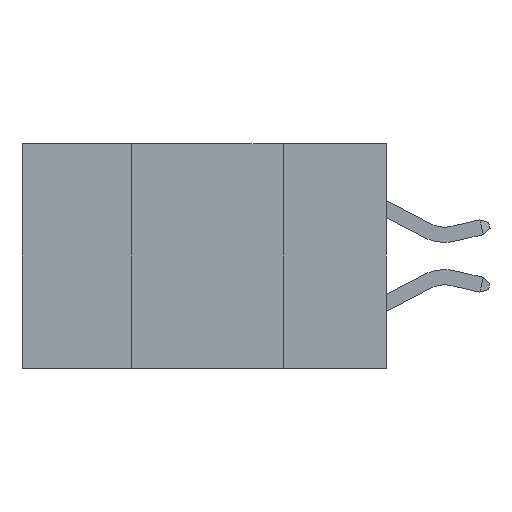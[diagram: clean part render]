
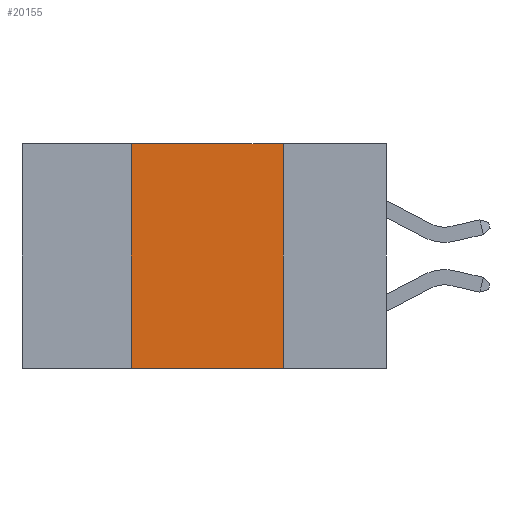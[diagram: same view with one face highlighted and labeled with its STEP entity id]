
A CAD part, left-side view. The second image highlights one B-rep face of the part: STEP entity #20155.
In plain terms, the highlighted planar face has unit normal (-1, 0, 0).
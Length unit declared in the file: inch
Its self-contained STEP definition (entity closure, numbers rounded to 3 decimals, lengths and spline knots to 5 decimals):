
#507 = VERTEX_POINT ( 'NONE', #6065 ) ;
#593 = VECTOR ( 'NONE', #23054, 39.37008 ) ;
#1452 = CARTESIAN_POINT ( 'NONE',  ( 0., 0.6, 0. ) ) ;
#3165 = AXIS2_PLACEMENT_3D ( 'NONE', #1452, #18680, #3948 ) ;
#3948 = DIRECTION ( 'NONE',  ( 0., 0., -1. ) ) ;
#4533 = EDGE_LOOP ( 'NONE', ( #10793, #12500, #26225, #17152 ) ) ;
#5935 = CARTESIAN_POINT ( 'NONE',  ( 0., 0.6, -0.37 ) ) ;
#6065 = CARTESIAN_POINT ( 'NONE',  ( 0., 0.17, 0. ) ) ;
#6295 = VECTOR ( 'NONE', #22303, 39.37008 ) ;
#8895 = EDGE_CURVE ( 'NONE', #11816, #22956, #18727, .T. ) ;
#9766 = VERTEX_POINT ( 'NONE', #12756 ) ;
#10793 = ORIENTED_EDGE ( 'NONE', *, *, #13253, .F. ) ;
#10853 = LINE ( 'NONE', #24334, #29440 ) ;
#11816 = VERTEX_POINT ( 'NONE', #22746 ) ;
#12500 = ORIENTED_EDGE ( 'NONE', *, *, #26338, .F. ) ;
#12756 = CARTESIAN_POINT ( 'NONE',  ( 0., 0.42, 0. ) ) ;
#13253 = EDGE_CURVE ( 'NONE', #507, #22956, #31416, .T. ) ;
#13889 = LINE ( 'NONE', #26819, #26776 ) ;
#14591 = DIRECTION ( 'NONE',  ( 0., 0., 1. ) ) ;
#15356 = CARTESIAN_POINT ( 'NONE',  ( 0., 0.17, -0.37 ) ) ;
#17130 = DIRECTION ( 'NONE',  ( 0., -1., 0. ) ) ;
#17152 = ORIENTED_EDGE ( 'NONE', *, *, #8895, .T. ) ;
#18680 = DIRECTION ( 'NONE',  ( 1., 0., 0. ) ) ;
#18727 = LINE ( 'NONE', #5935, #593 ) ;
#20155 = ADVANCED_FACE ( 'NONE', ( #27421 ), #28282, .F. ) ;
#22303 = DIRECTION ( 'NONE',  ( 0., 0., -1. ) ) ;
#22746 = CARTESIAN_POINT ( 'NONE',  ( 0., 0.42, -0.37 ) ) ;
#22956 = VERTEX_POINT ( 'NONE', #15356 ) ;
#23054 = DIRECTION ( 'NONE',  ( 0., -1., 0. ) ) ;
#24334 = CARTESIAN_POINT ( 'NONE',  ( 0., 0.42, 0. ) ) ;
#26225 = ORIENTED_EDGE ( 'NONE', *, *, #30660, .F. ) ;
#26338 = EDGE_CURVE ( 'NONE', #9766, #507, #13889, .T. ) ;
#26776 = VECTOR ( 'NONE', #17130, 39.37008 ) ;
#26819 = CARTESIAN_POINT ( 'NONE',  ( 0., 0.6, 0. ) ) ;
#27133 = CARTESIAN_POINT ( 'NONE',  ( 0., 0.17, 0. ) ) ;
#27421 = FACE_OUTER_BOUND ( 'NONE', #4533, .T. ) ;
#28282 = PLANE ( 'NONE',  #3165 ) ;
#29440 = VECTOR ( 'NONE', #14591, 39.37008 ) ;
#30660 = EDGE_CURVE ( 'NONE', #11816, #9766, #10853, .T. ) ;
#31416 = LINE ( 'NONE', #27133, #6295 ) ;
